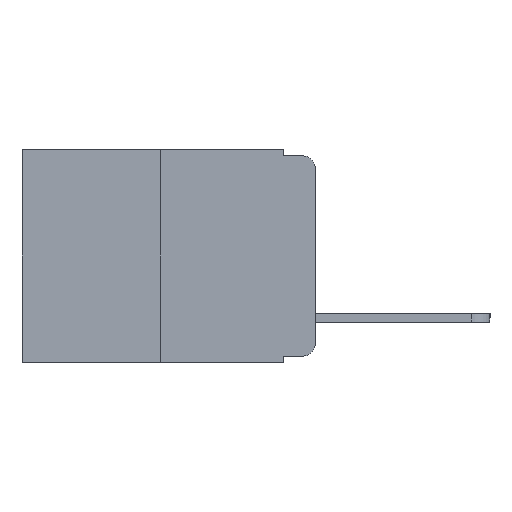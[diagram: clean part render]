
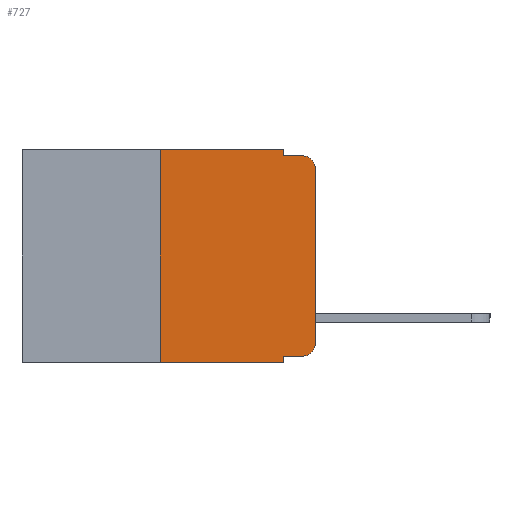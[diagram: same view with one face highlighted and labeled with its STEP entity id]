
A CAD part, left-side view. The second image highlights one B-rep face of the part: STEP entity #727.
In plain terms, the highlighted planar face has unit normal (-1, 0, 0).
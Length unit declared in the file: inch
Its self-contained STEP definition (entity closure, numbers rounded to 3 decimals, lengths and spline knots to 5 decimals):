
#53 = CARTESIAN_POINT ( 'NONE',  ( 0., 0.25, 0. ) ) ;
#242 = CARTESIAN_POINT ( 'NONE',  ( 0., 0.02, -0.03 ) ) ;
#526 = VERTEX_POINT ( 'NONE', #15852 ) ;
#554 = VERTEX_POINT ( 'NONE', #4100 ) ;
#576 = EDGE_CURVE ( 'NONE', #12371, #3145, #9405, .T. ) ;
#665 = DIRECTION ( 'NONE',  ( 0., 0., -1. ) ) ;
#727 = ADVANCED_FACE ( 'NONE', ( #10016 ), #2613, .F. ) ;
#1037 = DIRECTION ( 'NONE',  ( 0., -1., 0. ) ) ;
#1077 = CARTESIAN_POINT ( 'NONE',  ( 0., 0.473, 0. ) ) ;
#1618 = EDGE_CURVE ( 'NONE', #3145, #6837, #11593, .T. ) ;
#1803 = DIRECTION ( 'NONE',  ( 0., 0., -1. ) ) ;
#1943 = CARTESIAN_POINT ( 'NONE',  ( 0., 0.051, -0.343 ) ) ;
#1974 = CARTESIAN_POINT ( 'NONE',  ( 0., 0.25, 0. ) ) ;
#2169 = LINE ( 'NONE', #16427, #5042 ) ;
#2499 = VERTEX_POINT ( 'NONE', #1943 ) ;
#2510 = CARTESIAN_POINT ( 'NONE',  ( 0., 0.051, -0.01 ) ) ;
#2613 = PLANE ( 'NONE',  #10531 ) ;
#2951 = ORIENTED_EDGE ( 'NONE', *, *, #16850, .F. ) ;
#3145 = VERTEX_POINT ( 'NONE', #3447 ) ;
#3447 = CARTESIAN_POINT ( 'NONE',  ( 0., 0.051, -0.01 ) ) ;
#3580 = DIRECTION ( 'NONE',  ( 0., 0., 1. ) ) ;
#3607 = EDGE_CURVE ( 'NONE', #5858, #6837, #4649, .T. ) ;
#3637 = ORIENTED_EDGE ( 'NONE', *, *, #7818, .T. ) ;
#4063 = DIRECTION ( 'NONE',  ( 1., 0., 0. ) ) ;
#4088 = LINE ( 'NONE', #1974, #11175 ) ;
#4100 = CARTESIAN_POINT ( 'NONE',  ( 0., 0.25, -0.343 ) ) ;
#4528 = EDGE_CURVE ( 'NONE', #8942, #5858, #2169, .T. ) ;
#4616 = DIRECTION ( 'NONE',  ( 0., -1., 0. ) ) ;
#4649 = CIRCLE ( 'NONE', #13851, 0.02 ) ;
#5042 = VECTOR ( 'NONE', #3580, 39.37008 ) ;
#5218 = EDGE_LOOP ( 'NONE', ( #12529, #11304, #13305, #13707, #15201, #2951, #3637, #13529, #9118, #9528 ) ) ;
#5858 = VERTEX_POINT ( 'NONE', #15092 ) ;
#5880 = VECTOR ( 'NONE', #10075, 39.37008 ) ;
#6051 = VECTOR ( 'NONE', #4616, 39.37008 ) ;
#6322 = CARTESIAN_POINT ( 'NONE',  ( 0., 0.051, 0. ) ) ;
#6582 = CARTESIAN_POINT ( 'NONE',  ( 0., 0.051, -0.333 ) ) ;
#6837 = VERTEX_POINT ( 'NONE', #11874 ) ;
#7120 = VERTEX_POINT ( 'NONE', #53 ) ;
#7177 = EDGE_CURVE ( 'NONE', #7120, #12371, #9570, .T. ) ;
#7233 = CARTESIAN_POINT ( 'NONE',  ( 0., 0.473, -0.343 ) ) ;
#7500 = LINE ( 'NONE', #7233, #13934 ) ;
#7818 = EDGE_CURVE ( 'NONE', #554, #2499, #7500, .T. ) ;
#8627 = AXIS2_PLACEMENT_3D ( 'NONE', #16512, #9030, #665 ) ;
#8643 = VECTOR ( 'NONE', #11787, 39.37008 ) ;
#8942 = VERTEX_POINT ( 'NONE', #13521 ) ;
#9030 = DIRECTION ( 'NONE',  ( -1., 0., 0. ) ) ;
#9118 = ORIENTED_EDGE ( 'NONE', *, *, #15247, .T. ) ;
#9405 = LINE ( 'NONE', #6322, #5880 ) ;
#9528 = ORIENTED_EDGE ( 'NONE', *, *, #14454, .T. ) ;
#9570 = LINE ( 'NONE', #12538, #6051 ) ;
#9889 = LINE ( 'NONE', #6582, #8643 ) ;
#10007 = DIRECTION ( 'NONE',  ( -1., 0., 0. ) ) ;
#10016 = FACE_OUTER_BOUND ( 'NONE', #5218, .T. ) ;
#10075 = DIRECTION ( 'NONE',  ( 0., 0., -1. ) ) ;
#10531 = AXIS2_PLACEMENT_3D ( 'NONE', #1077, #4063, #13252 ) ;
#11033 = DIRECTION ( 'NONE',  ( 0., 0., -1. ) ) ;
#11088 = CARTESIAN_POINT ( 'NONE',  ( 0., 0.051, 0. ) ) ;
#11175 = VECTOR ( 'NONE', #12696, 39.37008 ) ;
#11304 = ORIENTED_EDGE ( 'NONE', *, *, #3607, .T. ) ;
#11593 = LINE ( 'NONE', #2510, #15253 ) ;
#11787 = DIRECTION ( 'NONE',  ( 0., -1., 0. ) ) ;
#11874 = CARTESIAN_POINT ( 'NONE',  ( 0., 0.02, -0.01 ) ) ;
#11920 = CIRCLE ( 'NONE', #8627, 0.02 ) ;
#12185 = LINE ( 'NONE', #11088, #15418 ) ;
#12283 = CARTESIAN_POINT ( 'NONE',  ( 0., 0.051, 0. ) ) ;
#12371 = VERTEX_POINT ( 'NONE', #12283 ) ;
#12529 = ORIENTED_EDGE ( 'NONE', *, *, #4528, .T. ) ;
#12538 = CARTESIAN_POINT ( 'NONE',  ( 0., 0.473, 0. ) ) ;
#12696 = DIRECTION ( 'NONE',  ( 0., 0., 1. ) ) ;
#12703 = VERTEX_POINT ( 'NONE', #15302 ) ;
#13252 = DIRECTION ( 'NONE',  ( 0., 0., -1. ) ) ;
#13305 = ORIENTED_EDGE ( 'NONE', *, *, #1618, .F. ) ;
#13521 = CARTESIAN_POINT ( 'NONE',  ( 0., 0., -0.313 ) ) ;
#13529 = ORIENTED_EDGE ( 'NONE', *, *, #16040, .F. ) ;
#13707 = ORIENTED_EDGE ( 'NONE', *, *, #576, .F. ) ;
#13851 = AXIS2_PLACEMENT_3D ( 'NONE', #242, #10007, #1803 ) ;
#13934 = VECTOR ( 'NONE', #14869, 39.37008 ) ;
#14454 = EDGE_CURVE ( 'NONE', #12703, #8942, #11920, .T. ) ;
#14869 = DIRECTION ( 'NONE',  ( 0., -1., 0. ) ) ;
#15092 = CARTESIAN_POINT ( 'NONE',  ( 0., 0., -0.03 ) ) ;
#15201 = ORIENTED_EDGE ( 'NONE', *, *, #7177, .F. ) ;
#15247 = EDGE_CURVE ( 'NONE', #526, #12703, #9889, .T. ) ;
#15253 = VECTOR ( 'NONE', #1037, 39.37008 ) ;
#15302 = CARTESIAN_POINT ( 'NONE',  ( 0., 0.02, -0.333 ) ) ;
#15418 = VECTOR ( 'NONE', #11033, 39.37008 ) ;
#15852 = CARTESIAN_POINT ( 'NONE',  ( 0., 0.051, -0.333 ) ) ;
#16040 = EDGE_CURVE ( 'NONE', #526, #2499, #12185, .T. ) ;
#16427 = CARTESIAN_POINT ( 'NONE',  ( 0., 0., 0. ) ) ;
#16512 = CARTESIAN_POINT ( 'NONE',  ( 0., 0.02, -0.313 ) ) ;
#16850 = EDGE_CURVE ( 'NONE', #554, #7120, #4088, .T. ) ;
